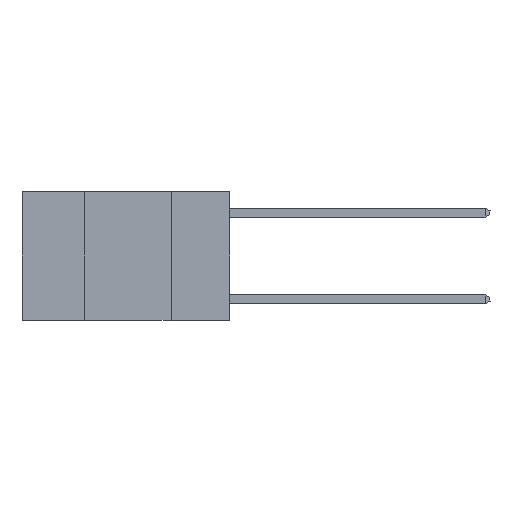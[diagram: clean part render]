
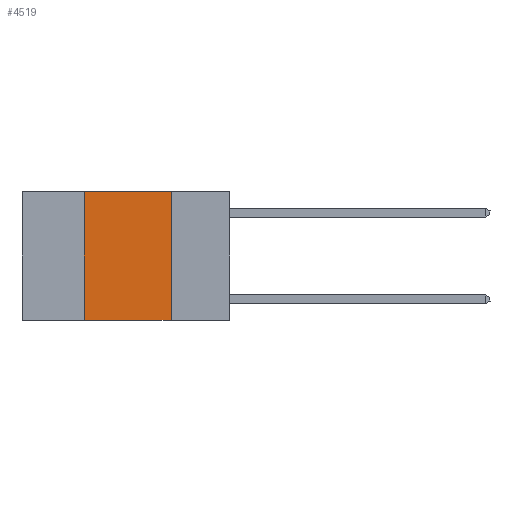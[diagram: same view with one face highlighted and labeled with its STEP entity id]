
A CAD part, left-side view. The second image highlights one B-rep face of the part: STEP entity #4519.
In plain terms, the highlighted planar face has unit normal (-1, 0, 0).
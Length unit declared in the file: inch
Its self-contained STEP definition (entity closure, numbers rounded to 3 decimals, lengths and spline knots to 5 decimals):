
#245 = LINE ( 'NONE', #20726, #10992 ) ;
#2115 = CARTESIAN_POINT ( 'NONE',  ( 0., 0.17, 0. ) ) ;
#2230 = CARTESIAN_POINT ( 'NONE',  ( 0., 0.6, -0.37 ) ) ;
#3628 = CARTESIAN_POINT ( 'NONE',  ( 0., 0.42, 0. ) ) ;
#4519 = ADVANCED_FACE ( 'NONE', ( #26987 ), #24742, .F. ) ;
#4804 = VERTEX_POINT ( 'NONE', #14637 ) ;
#6326 = LINE ( 'NONE', #3628, #8393 ) ;
#8132 = DIRECTION ( 'NONE',  ( 0., 0., 1. ) ) ;
#8393 = VECTOR ( 'NONE', #8132, 39.37008 ) ;
#8397 = ORIENTED_EDGE ( 'NONE', *, *, #11873, .F. ) ;
#8648 = EDGE_CURVE ( 'NONE', #27042, #4804, #8851, .T. ) ;
#8851 = LINE ( 'NONE', #2115, #28477 ) ;
#9339 = EDGE_CURVE ( 'NONE', #15816, #4804, #25148, .T. ) ;
#10028 = CARTESIAN_POINT ( 'NONE',  ( 0., 0.42, 0. ) ) ;
#10510 = CARTESIAN_POINT ( 'NONE',  ( 0., 0.6, 0. ) ) ;
#10646 = DIRECTION ( 'NONE',  ( 0., 0., -1. ) ) ;
#10992 = VECTOR ( 'NONE', #27213, 39.37008 ) ;
#11356 = DIRECTION ( 'NONE',  ( 0., -1., 0. ) ) ;
#11873 = EDGE_CURVE ( 'NONE', #15816, #18935, #6326, .T. ) ;
#12963 = CARTESIAN_POINT ( 'NONE',  ( 0., 0.42, -0.37 ) ) ;
#13351 = CARTESIAN_POINT ( 'NONE',  ( 0., 0.17, 0. ) ) ;
#13357 = DIRECTION ( 'NONE',  ( 1., 0., 0. ) ) ;
#13687 = ORIENTED_EDGE ( 'NONE', *, *, #9339, .T. ) ;
#14637 = CARTESIAN_POINT ( 'NONE',  ( 0., 0.17, -0.37 ) ) ;
#15816 = VERTEX_POINT ( 'NONE', #12963 ) ;
#18935 = VERTEX_POINT ( 'NONE', #10028 ) ;
#19355 = EDGE_CURVE ( 'NONE', #18935, #27042, #245, .T. ) ;
#19612 = DIRECTION ( 'NONE',  ( 0., 0., -1. ) ) ;
#20204 = AXIS2_PLACEMENT_3D ( 'NONE', #10510, #13357, #19612 ) ;
#20726 = CARTESIAN_POINT ( 'NONE',  ( 0., 0.6, 0. ) ) ;
#21638 = VECTOR ( 'NONE', #11356, 39.37008 ) ;
#23056 = ORIENTED_EDGE ( 'NONE', *, *, #19355, .F. ) ;
#24281 = ORIENTED_EDGE ( 'NONE', *, *, #8648, .F. ) ;
#24742 = PLANE ( 'NONE',  #20204 ) ;
#25148 = LINE ( 'NONE', #2230, #21638 ) ;
#26256 = EDGE_LOOP ( 'NONE', ( #24281, #23056, #8397, #13687 ) ) ;
#26987 = FACE_OUTER_BOUND ( 'NONE', #26256, .T. ) ;
#27042 = VERTEX_POINT ( 'NONE', #13351 ) ;
#27213 = DIRECTION ( 'NONE',  ( 0., -1., 0. ) ) ;
#28477 = VECTOR ( 'NONE', #10646, 39.37008 ) ;
